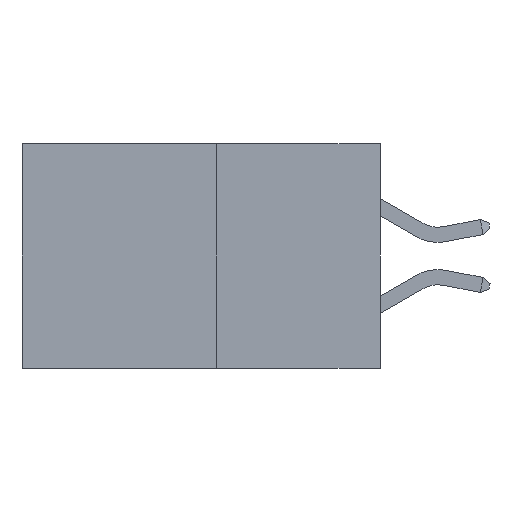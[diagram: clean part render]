
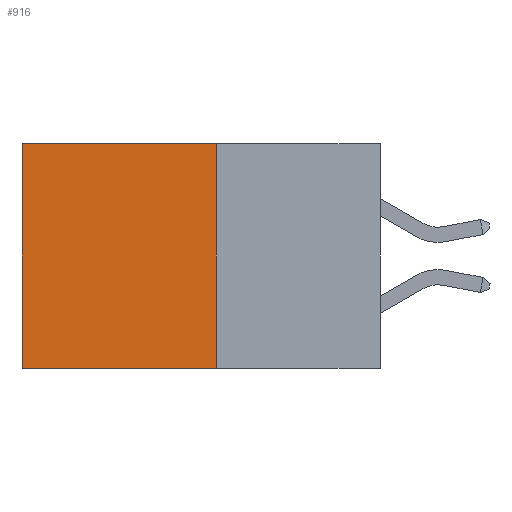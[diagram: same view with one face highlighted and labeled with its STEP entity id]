
A CAD part, left-side view. The second image highlights one B-rep face of the part: STEP entity #916.
In plain terms, the highlighted planar face has unit normal (-1, 0, 0).
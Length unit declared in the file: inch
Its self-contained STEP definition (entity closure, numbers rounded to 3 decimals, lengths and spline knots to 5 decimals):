
#83 = VERTEX_POINT ( 'NONE', #13982 ) ;
#754 = VERTEX_POINT ( 'NONE', #1483 ) ;
#829 = EDGE_CURVE ( 'NONE', #15219, #4607, #8930, .T. ) ;
#916 = ADVANCED_FACE ( 'NONE', ( #15033 ), #12895, .F. ) ;
#1483 = CARTESIAN_POINT ( 'NONE',  ( 0.277, 0.27, 0. ) ) ;
#1761 = ORIENTED_EDGE ( 'NONE', *, *, #16457, .T. ) ;
#2900 = DIRECTION ( 'NONE',  ( 0., 1., 0. ) ) ;
#2943 = CARTESIAN_POINT ( 'NONE',  ( 0.277, 0.59, -0.37 ) ) ;
#3162 = ORIENTED_EDGE ( 'NONE', *, *, #10851, .F. ) ;
#3967 = EDGE_LOOP ( 'NONE', ( #1761, #5742, #3162, #17514 ) ) ;
#4571 = AXIS2_PLACEMENT_3D ( 'NONE', #12685, #12609, #12486 ) ;
#4607 = VERTEX_POINT ( 'NONE', #13834 ) ;
#4630 = LINE ( 'NONE', #7045, #11606 ) ;
#5742 = ORIENTED_EDGE ( 'NONE', *, *, #829, .F. ) ;
#7045 = CARTESIAN_POINT ( 'NONE',  ( 0.277, 0.27, 0. ) ) ;
#7842 = CARTESIAN_POINT ( 'NONE',  ( 0.277, 0.27, -0.37 ) ) ;
#8930 = LINE ( 'NONE', #16625, #12657 ) ;
#10851 = EDGE_CURVE ( 'NONE', #754, #15219, #16579, .T. ) ;
#11399 = CARTESIAN_POINT ( 'NONE',  ( 0.277, 0.27, -0.37 ) ) ;
#11606 = VECTOR ( 'NONE', #2900, 39.37008 ) ;
#11789 = VECTOR ( 'NONE', #14077, 39.37008 ) ;
#12486 = DIRECTION ( 'NONE',  ( 0., 0., -1. ) ) ;
#12609 = DIRECTION ( 'NONE',  ( 1., 0., 0. ) ) ;
#12657 = VECTOR ( 'NONE', #16744, 39.37008 ) ;
#12685 = CARTESIAN_POINT ( 'NONE',  ( 0.277, 0.27, -0.37 ) ) ;
#12895 = PLANE ( 'NONE',  #4571 ) ;
#12945 = VECTOR ( 'NONE', #17588, 39.37008 ) ;
#13834 = CARTESIAN_POINT ( 'NONE',  ( 0.277, 0.59, -0.37 ) ) ;
#13982 = CARTESIAN_POINT ( 'NONE',  ( 0.277, 0.59, 0. ) ) ;
#14077 = DIRECTION ( 'NONE',  ( 0., 0., -1. ) ) ;
#15033 = FACE_OUTER_BOUND ( 'NONE', #3967, .T. ) ;
#15219 = VERTEX_POINT ( 'NONE', #11399 ) ;
#15461 = LINE ( 'NONE', #2943, #11789 ) ;
#15797 = EDGE_CURVE ( 'NONE', #754, #83, #4630, .T. ) ;
#16457 = EDGE_CURVE ( 'NONE', #83, #4607, #15461, .T. ) ;
#16579 = LINE ( 'NONE', #7842, #12945 ) ;
#16625 = CARTESIAN_POINT ( 'NONE',  ( 0.277, 0.27, -0.37 ) ) ;
#16744 = DIRECTION ( 'NONE',  ( 0., 1., 0. ) ) ;
#17514 = ORIENTED_EDGE ( 'NONE', *, *, #15797, .T. ) ;
#17588 = DIRECTION ( 'NONE',  ( 0., 0., -1. ) ) ;
